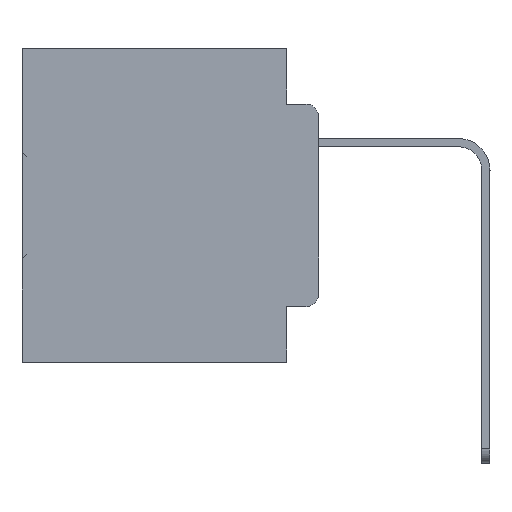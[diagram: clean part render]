
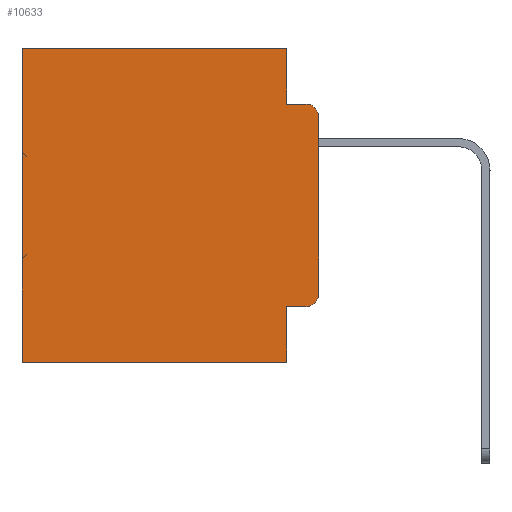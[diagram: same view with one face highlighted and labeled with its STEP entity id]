
A CAD part, left-side view. The second image highlights one B-rep face of the part: STEP entity #10633.
In plain terms, the highlighted planar face has unit normal (-1, 0, 0).
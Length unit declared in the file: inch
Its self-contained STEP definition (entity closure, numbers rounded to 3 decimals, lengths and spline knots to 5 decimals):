
#283 = CARTESIAN_POINT ( 'NONE',  ( 0.298, 0.02, -0.3915 ) ) ;
#375 = AXIS2_PLACEMENT_3D ( 'NONE', #283, #8473, #401 ) ;
#401 = DIRECTION ( 'NONE',  ( 0., 0., -1. ) ) ;
#419 = DIRECTION ( 'NONE',  ( 0., 0., -1. ) ) ;
#727 = CARTESIAN_POINT ( 'NONE',  ( 0.298, 0.051, -0.0885 ) ) ;
#1496 = VERTEX_POINT ( 'NONE', #25865 ) ;
#1755 = CIRCLE ( 'NONE', #375, 0.02 ) ;
#2019 = CARTESIAN_POINT ( 'NONE',  ( 0.298, 0.051, -0.5 ) ) ;
#2095 = VERTEX_POINT ( 'NONE', #3155 ) ;
#2576 = ORIENTED_EDGE ( 'NONE', *, *, #11964, .T. ) ;
#3155 = CARTESIAN_POINT ( 'NONE',  ( 0.298, 0.473, 0. ) ) ;
#3252 = CARTESIAN_POINT ( 'NONE',  ( 0.298, 0., -0.1085 ) ) ;
#3366 = FACE_OUTER_BOUND ( 'NONE', #23195, .T. ) ;
#3563 = EDGE_CURVE ( 'NONE', #23568, #13578, #16378, .T. ) ;
#3915 = CARTESIAN_POINT ( 'NONE',  ( 0.298, 0.02, -0.1085 ) ) ;
#4466 = VECTOR ( 'NONE', #10970, 39.37008 ) ;
#4668 = ORIENTED_EDGE ( 'NONE', *, *, #16668, .F. ) ;
#6944 = LINE ( 'NONE', #11726, #10772 ) ;
#7467 = DIRECTION ( 'NONE',  ( 0., -1., 0. ) ) ;
#7843 = LINE ( 'NONE', #19790, #15885 ) ;
#8473 = DIRECTION ( 'NONE',  ( -1., 0., 0. ) ) ;
#8512 = LINE ( 'NONE', #12800, #34721 ) ;
#8605 = EDGE_CURVE ( 'NONE', #22215, #13578, #1755, .T. ) ;
#8608 = CARTESIAN_POINT ( 'NONE',  ( 0.298, 0., 0. ) ) ;
#9341 = ORIENTED_EDGE ( 'NONE', *, *, #12455, .F. ) ;
#9545 = CARTESIAN_POINT ( 'NONE',  ( 0.298, 0., -0.5 ) ) ;
#10631 = CARTESIAN_POINT ( 'NONE',  ( 0.298, 0., -0.3915 ) ) ;
#10633 = ADVANCED_FACE ( 'NONE', ( #3366 ), #24299, .F. ) ;
#10772 = VECTOR ( 'NONE', #30641, 39.37008 ) ;
#10959 = DIRECTION ( 'NONE',  ( 1., 0., 0. ) ) ;
#10970 = DIRECTION ( 'NONE',  ( 0., 0., -1. ) ) ;
#11276 = DIRECTION ( 'NONE',  ( 0., -1., 0. ) ) ;
#11590 = VERTEX_POINT ( 'NONE', #28766 ) ;
#11726 = CARTESIAN_POINT ( 'NONE',  ( 0.298, 0.473, 0. ) ) ;
#11964 = EDGE_CURVE ( 'NONE', #23568, #21462, #33693, .T. ) ;
#12092 = CARTESIAN_POINT ( 'NONE',  ( 0.298, 0.02, -0.0885 ) ) ;
#12455 = EDGE_CURVE ( 'NONE', #1496, #32632, #29436, .T. ) ;
#12800 = CARTESIAN_POINT ( 'NONE',  ( 0.298, 0.051, -0.4115 ) ) ;
#12831 = CARTESIAN_POINT ( 'NONE',  ( 0.298, 0.473, -0.5 ) ) ;
#13578 = VERTEX_POINT ( 'NONE', #10631 ) ;
#14062 = ORIENTED_EDGE ( 'NONE', *, *, #33501, .T. ) ;
#15885 = VECTOR ( 'NONE', #25249, 39.37008 ) ;
#16270 = DIRECTION ( 'NONE',  ( 0., 1., 0. ) ) ;
#16378 = LINE ( 'NONE', #8608, #29912 ) ;
#16668 = EDGE_CURVE ( 'NONE', #32632, #21462, #35111, .T. ) ;
#16795 = CARTESIAN_POINT ( 'NONE',  ( 0.298, 0.02, -0.4115 ) ) ;
#17257 = DIRECTION ( 'NONE',  ( -1., 0., 0. ) ) ;
#17440 = AXIS2_PLACEMENT_3D ( 'NONE', #21782, #10959, #32698 ) ;
#18963 = CARTESIAN_POINT ( 'NONE',  ( 0.298, 0., 0. ) ) ;
#19027 = AXIS2_PLACEMENT_3D ( 'NONE', #3915, #17257, #22427 ) ;
#19790 = CARTESIAN_POINT ( 'NONE',  ( 0.298, 0.051, 0. ) ) ;
#21462 = VERTEX_POINT ( 'NONE', #12092 ) ;
#21782 = CARTESIAN_POINT ( 'NONE',  ( 0.298, 0., 0. ) ) ;
#22215 = VERTEX_POINT ( 'NONE', #16795 ) ;
#22427 = DIRECTION ( 'NONE',  ( 0., 0., -1. ) ) ;
#22974 = ORIENTED_EDGE ( 'NONE', *, *, #8605, .T. ) ;
#23165 = EDGE_CURVE ( 'NONE', #11590, #31186, #7843, .T. ) ;
#23195 = EDGE_LOOP ( 'NONE', ( #30907, #2576, #4668, #9341, #27704, #33645, #32537, #26554, #14062, #22974 ) ) ;
#23568 = VERTEX_POINT ( 'NONE', #3252 ) ;
#24299 = PLANE ( 'NONE',  #17440 ) ;
#25249 = DIRECTION ( 'NONE',  ( 0., 0., -1. ) ) ;
#25865 = CARTESIAN_POINT ( 'NONE',  ( 0.298, 0.051, 0. ) ) ;
#26554 = ORIENTED_EDGE ( 'NONE', *, *, #23165, .F. ) ;
#26642 = LINE ( 'NONE', #9545, #28790 ) ;
#27183 = CARTESIAN_POINT ( 'NONE',  ( 0.298, 0.051, 0. ) ) ;
#27491 = CARTESIAN_POINT ( 'NONE',  ( 0.298, 0.051, -0.0885 ) ) ;
#27704 = ORIENTED_EDGE ( 'NONE', *, *, #28351, .T. ) ;
#27951 = VECTOR ( 'NONE', #11276, 39.37008 ) ;
#28152 = EDGE_CURVE ( 'NONE', #31186, #31665, #26642, .T. ) ;
#28351 = EDGE_CURVE ( 'NONE', #1496, #2095, #34235, .T. ) ;
#28766 = CARTESIAN_POINT ( 'NONE',  ( 0.298, 0.051, -0.4115 ) ) ;
#28790 = VECTOR ( 'NONE', #31162, 39.37008 ) ;
#29436 = LINE ( 'NONE', #27183, #4466 ) ;
#29912 = VECTOR ( 'NONE', #419, 39.37008 ) ;
#30641 = DIRECTION ( 'NONE',  ( 0., 0., -1. ) ) ;
#30907 = ORIENTED_EDGE ( 'NONE', *, *, #3563, .F. ) ;
#30935 = EDGE_CURVE ( 'NONE', #2095, #31665, #6944, .T. ) ;
#31162 = DIRECTION ( 'NONE',  ( 0., 1., 0. ) ) ;
#31186 = VERTEX_POINT ( 'NONE', #2019 ) ;
#31269 = VECTOR ( 'NONE', #16270, 39.37008 ) ;
#31665 = VERTEX_POINT ( 'NONE', #12831 ) ;
#32537 = ORIENTED_EDGE ( 'NONE', *, *, #28152, .F. ) ;
#32632 = VERTEX_POINT ( 'NONE', #727 ) ;
#32698 = DIRECTION ( 'NONE',  ( 0., 0., -1. ) ) ;
#33501 = EDGE_CURVE ( 'NONE', #11590, #22215, #8512, .T. ) ;
#33645 = ORIENTED_EDGE ( 'NONE', *, *, #30935, .T. ) ;
#33693 = CIRCLE ( 'NONE', #19027, 0.02 ) ;
#34235 = LINE ( 'NONE', #18963, #31269 ) ;
#34721 = VECTOR ( 'NONE', #7467, 39.37008 ) ;
#35111 = LINE ( 'NONE', #27491, #27951 ) ;
